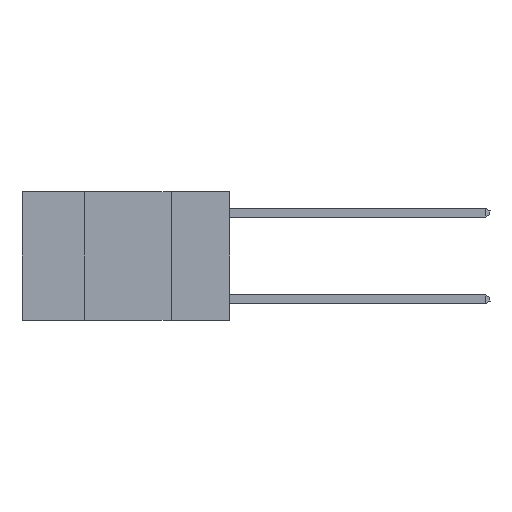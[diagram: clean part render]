
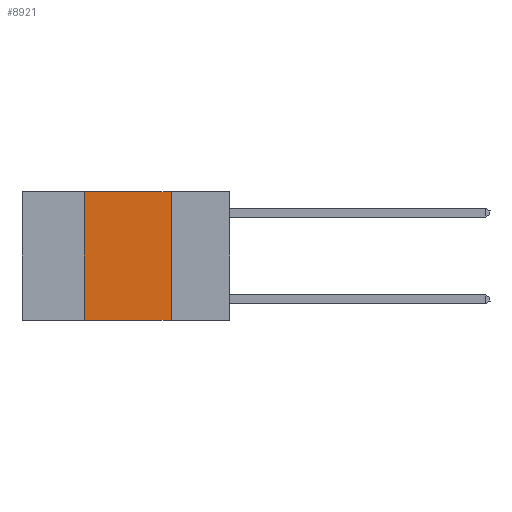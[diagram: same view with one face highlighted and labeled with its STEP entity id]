
A CAD part, left-side view. The second image highlights one B-rep face of the part: STEP entity #8921.
In plain terms, the highlighted planar face has unit normal (-1, 0, 0).
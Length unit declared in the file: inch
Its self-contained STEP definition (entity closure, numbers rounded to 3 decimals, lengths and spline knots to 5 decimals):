
#249 = CARTESIAN_POINT ( 'NONE',  ( 0., 0.17, 0. ) ) ;
#367 = CARTESIAN_POINT ( 'NONE',  ( 0., 0.42, 0. ) ) ;
#1591 = FACE_OUTER_BOUND ( 'NONE', #3844, .T. ) ;
#1935 = VECTOR ( 'NONE', #10996, 39.37008 ) ;
#2228 = LINE ( 'NONE', #367, #4007 ) ;
#2273 = ORIENTED_EDGE ( 'NONE', *, *, #11515, .F. ) ;
#2288 = AXIS2_PLACEMENT_3D ( 'NONE', #6293, #12084, #4267 ) ;
#2688 = CARTESIAN_POINT ( 'NONE',  ( 0., 0.6, -0.37 ) ) ;
#3844 = EDGE_LOOP ( 'NONE', ( #11193, #8082, #2273, #8482 ) ) ;
#4007 = VECTOR ( 'NONE', #11177, 39.37008 ) ;
#4008 = LINE ( 'NONE', #249, #1935 ) ;
#4267 = DIRECTION ( 'NONE',  ( 0., 0., -1. ) ) ;
#4619 = DIRECTION ( 'NONE',  ( 0., -1., 0. ) ) ;
#4730 = VERTEX_POINT ( 'NONE', #8017 ) ;
#6154 = VECTOR ( 'NONE', #6553, 39.37008 ) ;
#6293 = CARTESIAN_POINT ( 'NONE',  ( 0., 0.6, 0. ) ) ;
#6553 = DIRECTION ( 'NONE',  ( 0., -1., 0. ) ) ;
#6796 = VERTEX_POINT ( 'NONE', #11514 ) ;
#6952 = EDGE_CURVE ( 'NONE', #4730, #7086, #8387, .T. ) ;
#7086 = VERTEX_POINT ( 'NONE', #10450 ) ;
#7902 = CARTESIAN_POINT ( 'NONE',  ( 0., 0.17, 0. ) ) ;
#8017 = CARTESIAN_POINT ( 'NONE',  ( 0., 0.42, -0.37 ) ) ;
#8082 = ORIENTED_EDGE ( 'NONE', *, *, #10497, .F. ) ;
#8387 = LINE ( 'NONE', #2688, #6154 ) ;
#8482 = ORIENTED_EDGE ( 'NONE', *, *, #6952, .T. ) ;
#8921 = ADVANCED_FACE ( 'NONE', ( #1591 ), #9106, .F. ) ;
#9106 = PLANE ( 'NONE',  #2288 ) ;
#10450 = CARTESIAN_POINT ( 'NONE',  ( 0., 0.17, -0.37 ) ) ;
#10497 = EDGE_CURVE ( 'NONE', #6796, #11152, #12303, .T. ) ;
#10996 = DIRECTION ( 'NONE',  ( 0., 0., -1. ) ) ;
#11147 = EDGE_CURVE ( 'NONE', #11152, #7086, #4008, .T. ) ;
#11152 = VERTEX_POINT ( 'NONE', #7902 ) ;
#11177 = DIRECTION ( 'NONE',  ( 0., 0., 1. ) ) ;
#11193 = ORIENTED_EDGE ( 'NONE', *, *, #11147, .F. ) ;
#11514 = CARTESIAN_POINT ( 'NONE',  ( 0., 0.42, 0. ) ) ;
#11515 = EDGE_CURVE ( 'NONE', #4730, #6796, #2228, .T. ) ;
#11954 = VECTOR ( 'NONE', #4619, 39.37008 ) ;
#12084 = DIRECTION ( 'NONE',  ( 1., 0., 0. ) ) ;
#12167 = CARTESIAN_POINT ( 'NONE',  ( 0., 0.6, 0. ) ) ;
#12303 = LINE ( 'NONE', #12167, #11954 ) ;
